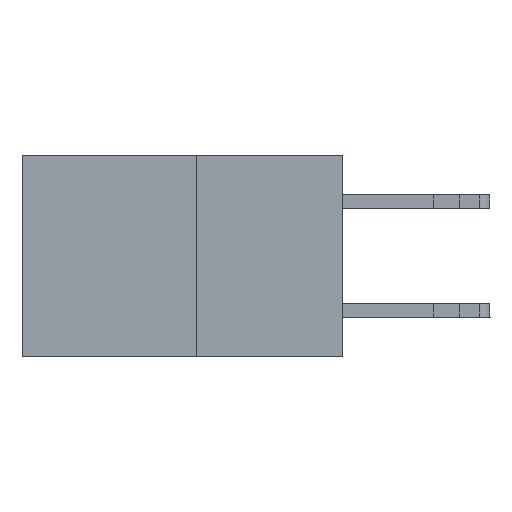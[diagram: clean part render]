
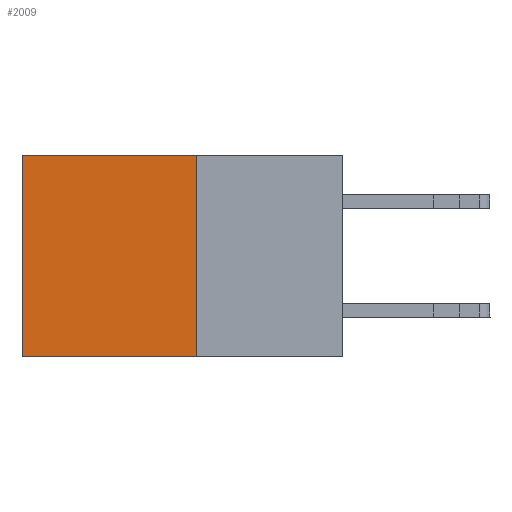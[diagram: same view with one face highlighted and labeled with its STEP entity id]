
A CAD part, left-side view. The second image highlights one B-rep face of the part: STEP entity #2009.
In plain terms, the highlighted planar face has unit normal (-1, 0, 0).
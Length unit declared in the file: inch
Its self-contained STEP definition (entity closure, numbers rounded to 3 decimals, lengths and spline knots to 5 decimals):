
#475 = ORIENTED_EDGE ( 'NONE', *, *, #3392, .T. ) ;
#1264 = LINE ( 'NONE', #7793, #6076 ) ;
#1516 = LINE ( 'NONE', #3614, #19734 ) ;
#1862 = VERTEX_POINT ( 'NONE', #8643 ) ;
#2009 = ADVANCED_FACE ( 'NONE', ( #3229 ), #12853, .F. ) ;
#2099 = LINE ( 'NONE', #8943, #6369 ) ;
#2476 = CARTESIAN_POINT ( 'NONE',  ( 0.277, 0.27, -0.37 ) ) ;
#3229 = FACE_OUTER_BOUND ( 'NONE', #20586, .T. ) ;
#3392 = EDGE_CURVE ( 'NONE', #1862, #5932, #10943, .T. ) ;
#3614 = CARTESIAN_POINT ( 'NONE',  ( 0.277, 0.59, -0.37 ) ) ;
#3660 = VERTEX_POINT ( 'NONE', #2476 ) ;
#5497 = DIRECTION ( 'NONE',  ( 0., 1., 0. ) ) ;
#5932 = VERTEX_POINT ( 'NONE', #15675 ) ;
#6052 = VERTEX_POINT ( 'NONE', #21276 ) ;
#6076 = VECTOR ( 'NONE', #9611, 39.37008 ) ;
#6369 = VECTOR ( 'NONE', #5497, 39.37008 ) ;
#7793 = CARTESIAN_POINT ( 'NONE',  ( 0.277, 0.27, -0.37 ) ) ;
#8643 = CARTESIAN_POINT ( 'NONE',  ( 0.277, 0.27, 0. ) ) ;
#8684 = EDGE_CURVE ( 'NONE', #5932, #6052, #1516, .T. ) ;
#8943 = CARTESIAN_POINT ( 'NONE',  ( 0.277, 0.27, -0.37 ) ) ;
#9611 = DIRECTION ( 'NONE',  ( 0., 0., -1. ) ) ;
#10052 = ORIENTED_EDGE ( 'NONE', *, *, #20978, .F. ) ;
#10943 = LINE ( 'NONE', #15345, #15047 ) ;
#12853 = PLANE ( 'NONE',  #17088 ) ;
#13229 = CARTESIAN_POINT ( 'NONE',  ( 0.277, 0.27, -0.37 ) ) ;
#13359 = ORIENTED_EDGE ( 'NONE', *, *, #20717, .F. ) ;
#14786 = DIRECTION ( 'NONE',  ( 0., 1., 0. ) ) ;
#14933 = DIRECTION ( 'NONE',  ( 0., 0., -1. ) ) ;
#14986 = DIRECTION ( 'NONE',  ( 1., 0., 0. ) ) ;
#15047 = VECTOR ( 'NONE', #14786, 39.37008 ) ;
#15345 = CARTESIAN_POINT ( 'NONE',  ( 0.277, 0.27, 0. ) ) ;
#15673 = ORIENTED_EDGE ( 'NONE', *, *, #8684, .T. ) ;
#15675 = CARTESIAN_POINT ( 'NONE',  ( 0.277, 0.59, 0. ) ) ;
#15942 = DIRECTION ( 'NONE',  ( 0., 0., -1. ) ) ;
#17088 = AXIS2_PLACEMENT_3D ( 'NONE', #13229, #14986, #14933 ) ;
#19734 = VECTOR ( 'NONE', #15942, 39.37008 ) ;
#20586 = EDGE_LOOP ( 'NONE', ( #15673, #13359, #10052, #475 ) ) ;
#20717 = EDGE_CURVE ( 'NONE', #3660, #6052, #2099, .T. ) ;
#20978 = EDGE_CURVE ( 'NONE', #1862, #3660, #1264, .T. ) ;
#21276 = CARTESIAN_POINT ( 'NONE',  ( 0.277, 0.59, -0.37 ) ) ;
